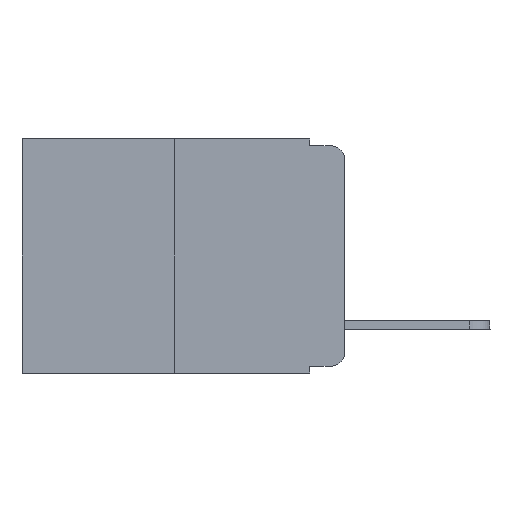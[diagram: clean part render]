
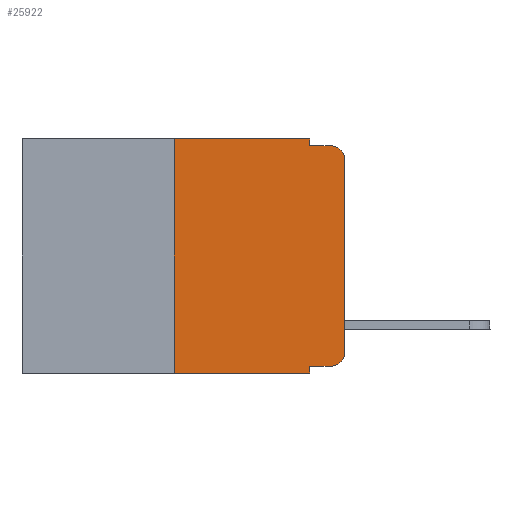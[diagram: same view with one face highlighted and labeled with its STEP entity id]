
A CAD part, left-side view. The second image highlights one B-rep face of the part: STEP entity #25922.
In plain terms, the highlighted planar face has unit normal (-1, 0, 0).
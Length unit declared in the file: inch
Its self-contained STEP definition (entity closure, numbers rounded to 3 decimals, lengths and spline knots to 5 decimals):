
#57 = CARTESIAN_POINT ( 'NONE',  ( 0., 0.473, -0.343 ) ) ;
#91 = LINE ( 'NONE', #6332, #17034 ) ;
#1231 = CARTESIAN_POINT ( 'NONE',  ( 0., 0.25, -0.343 ) ) ;
#1639 = VECTOR ( 'NONE', #25860, 39.37008 ) ;
#1820 = ORIENTED_EDGE ( 'NONE', *, *, #23705, .F. ) ;
#2131 = DIRECTION ( 'NONE',  ( 1., 0., 0. ) ) ;
#2277 = CARTESIAN_POINT ( 'NONE',  ( 0., 0.051, 0. ) ) ;
#2361 = DIRECTION ( 'NONE',  ( 0., -1., 0. ) ) ;
#3245 = EDGE_CURVE ( 'NONE', #5327, #21837, #12838, .T. ) ;
#3266 = ORIENTED_EDGE ( 'NONE', *, *, #3245, .T. ) ;
#3406 = DIRECTION ( 'NONE',  ( -1., 0., 0. ) ) ;
#3547 = CARTESIAN_POINT ( 'NONE',  ( 0., 0.051, -0.343 ) ) ;
#3627 = LINE ( 'NONE', #7343, #15458 ) ;
#3723 = CARTESIAN_POINT ( 'NONE',  ( 0., 0.051, -0.01 ) ) ;
#4174 = CARTESIAN_POINT ( 'NONE',  ( 0., 0.25, 0. ) ) ;
#4366 = CARTESIAN_POINT ( 'NONE',  ( 0., 0.02, -0.333 ) ) ;
#4471 = CARTESIAN_POINT ( 'NONE',  ( 0., 0.051, -0.333 ) ) ;
#4788 = EDGE_CURVE ( 'NONE', #21837, #18350, #3627, .T. ) ;
#4984 = CARTESIAN_POINT ( 'NONE',  ( 0., 0.051, -0.01 ) ) ;
#5098 = ORIENTED_EDGE ( 'NONE', *, *, #10792, .F. ) ;
#5327 = VERTEX_POINT ( 'NONE', #4366 ) ;
#5400 = LINE ( 'NONE', #57, #1639 ) ;
#6120 = VERTEX_POINT ( 'NONE', #15839 ) ;
#6332 = CARTESIAN_POINT ( 'NONE',  ( 0., 0.473, 0. ) ) ;
#6365 = CARTESIAN_POINT ( 'NONE',  ( 0., 0., -0.03 ) ) ;
#6499 = DIRECTION ( 'NONE',  ( 0., 0., -1. ) ) ;
#7011 = DIRECTION ( 'NONE',  ( -1., 0., 0. ) ) ;
#7262 = VERTEX_POINT ( 'NONE', #19065 ) ;
#7343 = CARTESIAN_POINT ( 'NONE',  ( 0., 0., 0. ) ) ;
#7768 = EDGE_LOOP ( 'NONE', ( #19656, #20991, #17534, #1820, #18627, #5098, #21782, #20913, #24538, #3266 ) ) ;
#8783 = CARTESIAN_POINT ( 'NONE',  ( 0., 0., -0.313 ) ) ;
#8803 = EDGE_CURVE ( 'NONE', #22290, #16355, #24321, .T. ) ;
#8999 = VECTOR ( 'NONE', #12266, 39.37008 ) ;
#9542 = LINE ( 'NONE', #17655, #12511 ) ;
#10093 = FACE_OUTER_BOUND ( 'NONE', #7768, .T. ) ;
#10792 = EDGE_CURVE ( 'NONE', #16619, #24927, #14245, .T. ) ;
#10981 = DIRECTION ( 'NONE',  ( 0., 0., -1. ) ) ;
#11633 = CARTESIAN_POINT ( 'NONE',  ( 0., 0.25, 0. ) ) ;
#11813 = DIRECTION ( 'NONE',  ( 0., -1., 0. ) ) ;
#12266 = DIRECTION ( 'NONE',  ( 0., 0., 1. ) ) ;
#12398 = EDGE_CURVE ( 'NONE', #18350, #6120, #16011, .T. ) ;
#12511 = VECTOR ( 'NONE', #15647, 39.37008 ) ;
#12582 = CARTESIAN_POINT ( 'NONE',  ( 0., 0.473, 0. ) ) ;
#12838 = CIRCLE ( 'NONE', #25159, 0.02 ) ;
#13306 = DIRECTION ( 'NONE',  ( 0., 0., 1. ) ) ;
#14245 = LINE ( 'NONE', #4174, #8999 ) ;
#14703 = CARTESIAN_POINT ( 'NONE',  ( 0., 0.051, -0.333 ) ) ;
#14704 = EDGE_CURVE ( 'NONE', #16619, #16355, #5400, .T. ) ;
#15458 = VECTOR ( 'NONE', #13306, 39.37008 ) ;
#15583 = AXIS2_PLACEMENT_3D ( 'NONE', #12582, #2131, #6499 ) ;
#15647 = DIRECTION ( 'NONE',  ( 0., 0., -1. ) ) ;
#15839 = CARTESIAN_POINT ( 'NONE',  ( 0., 0.02, -0.01 ) ) ;
#15866 = CARTESIAN_POINT ( 'NONE',  ( 0., 0.02, -0.03 ) ) ;
#16011 = CIRCLE ( 'NONE', #22818, 0.02 ) ;
#16355 = VERTEX_POINT ( 'NONE', #3547 ) ;
#16619 = VERTEX_POINT ( 'NONE', #1231 ) ;
#16894 = EDGE_CURVE ( 'NONE', #22853, #6120, #22303, .T. ) ;
#17034 = VECTOR ( 'NONE', #2361, 39.37008 ) ;
#17379 = CARTESIAN_POINT ( 'NONE',  ( 0., 0.02, -0.313 ) ) ;
#17514 = DIRECTION ( 'NONE',  ( 0., 0., -1. ) ) ;
#17534 = ORIENTED_EDGE ( 'NONE', *, *, #16894, .F. ) ;
#17655 = CARTESIAN_POINT ( 'NONE',  ( 0., 0.051, 0. ) ) ;
#18331 = PLANE ( 'NONE',  #15583 ) ;
#18350 = VERTEX_POINT ( 'NONE', #6365 ) ;
#18627 = ORIENTED_EDGE ( 'NONE', *, *, #18797, .F. ) ;
#18797 = EDGE_CURVE ( 'NONE', #24927, #7262, #91, .T. ) ;
#19065 = CARTESIAN_POINT ( 'NONE',  ( 0., 0.051, 0. ) ) ;
#19656 = ORIENTED_EDGE ( 'NONE', *, *, #4788, .T. ) ;
#19983 = DIRECTION ( 'NONE',  ( 0., 0., -1. ) ) ;
#20883 = VECTOR ( 'NONE', #20936, 39.37008 ) ;
#20913 = ORIENTED_EDGE ( 'NONE', *, *, #8803, .F. ) ;
#20936 = DIRECTION ( 'NONE',  ( 0., -1., 0. ) ) ;
#20991 = ORIENTED_EDGE ( 'NONE', *, *, #12398, .T. ) ;
#21398 = EDGE_CURVE ( 'NONE', #22290, #5327, #24668, .T. ) ;
#21606 = VECTOR ( 'NONE', #11813, 39.37008 ) ;
#21782 = ORIENTED_EDGE ( 'NONE', *, *, #14704, .T. ) ;
#21837 = VERTEX_POINT ( 'NONE', #8783 ) ;
#22290 = VERTEX_POINT ( 'NONE', #14703 ) ;
#22303 = LINE ( 'NONE', #3723, #21606 ) ;
#22818 = AXIS2_PLACEMENT_3D ( 'NONE', #15866, #3406, #19983 ) ;
#22853 = VERTEX_POINT ( 'NONE', #4984 ) ;
#23705 = EDGE_CURVE ( 'NONE', #7262, #22853, #9542, .T. ) ;
#23762 = VECTOR ( 'NONE', #10981, 39.37008 ) ;
#24321 = LINE ( 'NONE', #2277, #23762 ) ;
#24538 = ORIENTED_EDGE ( 'NONE', *, *, #21398, .T. ) ;
#24668 = LINE ( 'NONE', #4471, #20883 ) ;
#24927 = VERTEX_POINT ( 'NONE', #11633 ) ;
#25159 = AXIS2_PLACEMENT_3D ( 'NONE', #17379, #7011, #17514 ) ;
#25860 = DIRECTION ( 'NONE',  ( 0., -1., 0. ) ) ;
#25922 = ADVANCED_FACE ( 'NONE', ( #10093 ), #18331, .F. ) ;
